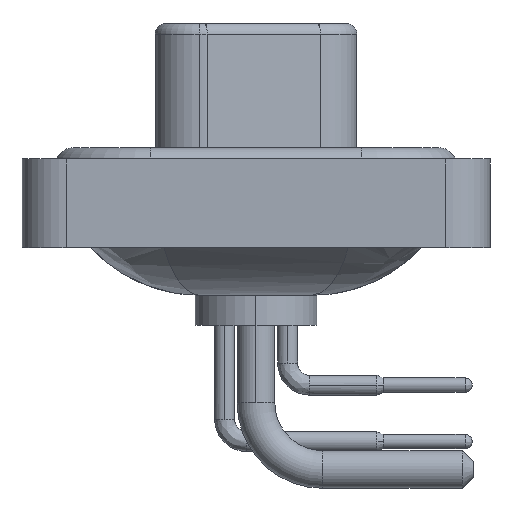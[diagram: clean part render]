
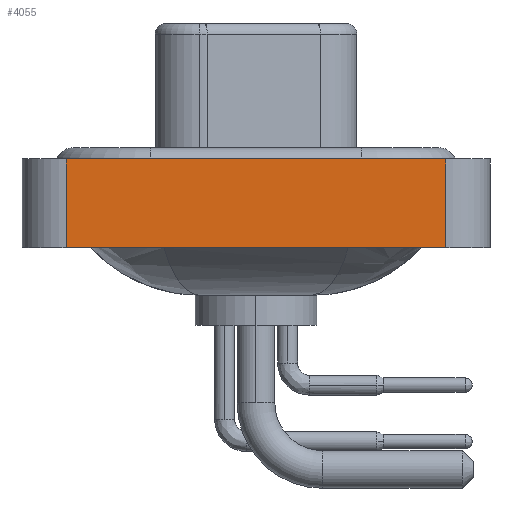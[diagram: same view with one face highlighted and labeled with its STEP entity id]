
A CAD part, left-side view. The second image highlights one B-rep face of the part: STEP entity #4055.
In plain terms, the highlighted planar face has unit normal (-1, 0, 0).
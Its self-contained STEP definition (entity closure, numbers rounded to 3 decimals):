
#981 = ORIENTED_EDGE ( 'NONE', *, *, #16964, .T. ) ;
#1514 = CARTESIAN_POINT ( 'NONE',  ( -7.35, -8.55, 0.4 ) ) ;
#2438 = ORIENTED_EDGE ( 'NONE', *, *, #9749, .F. ) ;
#3186 = AXIS2_PLACEMENT_3D ( 'NONE', #9276, #24573, #4792 ) ;
#3331 = DIRECTION ( 'NONE',  ( 0., 0., 1. ) ) ;
#3535 = EDGE_LOOP ( 'NONE', ( #981, #2438, #14370, #17733 ) ) ;
#4055 = ADVANCED_FACE ( 'NONE', ( #9128 ), #15759, .T. ) ;
#4123 = VECTOR ( 'NONE', #24071, 1000. ) ;
#4792 = DIRECTION ( 'NONE',  ( 0., 0., 1. ) ) ;
#4803 = EDGE_CURVE ( 'NONE', #16790, #16075, #14956, .T. ) ;
#5463 = CARTESIAN_POINT ( 'NONE',  ( -7.35, 8.55, -3.6 ) ) ;
#9128 = FACE_OUTER_BOUND ( 'NONE', #3535, .T. ) ;
#9276 = CARTESIAN_POINT ( 'NONE',  ( -7.35, -8.55, -3.6 ) ) ;
#9749 = EDGE_CURVE ( 'NONE', #14681, #9772, #12151, .T. ) ;
#9772 = VERTEX_POINT ( 'NONE', #11862 ) ;
#11862 = CARTESIAN_POINT ( 'NONE',  ( -7.35, -8.55, 0.4 ) ) ;
#12151 = LINE ( 'NONE', #1514, #17123 ) ;
#14370 = ORIENTED_EDGE ( 'NONE', *, *, #16257, .F. ) ;
#14681 = VERTEX_POINT ( 'NONE', #19489 ) ;
#14956 = LINE ( 'NONE', #15252, #4123 ) ;
#15029 = CARTESIAN_POINT ( 'NONE',  ( -7.35, -8.55, -3.6 ) ) ;
#15252 = CARTESIAN_POINT ( 'NONE',  ( -7.35, -8.55, -3.6 ) ) ;
#15508 = DIRECTION ( 'NONE',  ( 0., 0., 1. ) ) ;
#15759 = PLANE ( 'NONE',  #3186 ) ;
#16075 = VERTEX_POINT ( 'NONE', #15029 ) ;
#16257 = EDGE_CURVE ( 'NONE', #16790, #14681, #25246, .T. ) ;
#16790 = VERTEX_POINT ( 'NONE', #27802 ) ;
#16906 = DIRECTION ( 'NONE',  ( 0., -1., 0. ) ) ;
#16964 = EDGE_CURVE ( 'NONE', #16075, #9772, #26196, .T. ) ;
#17123 = VECTOR ( 'NONE', #16906, 1000. ) ;
#17733 = ORIENTED_EDGE ( 'NONE', *, *, #4803, .T. ) ;
#17964 = VECTOR ( 'NONE', #15508, 1000. ) ;
#19489 = CARTESIAN_POINT ( 'NONE',  ( -7.35, 8.55, 0.4 ) ) ;
#22984 = VECTOR ( 'NONE', #3331, 1000. ) ;
#24047 = CARTESIAN_POINT ( 'NONE',  ( -7.35, -8.55, -3.6 ) ) ;
#24071 = DIRECTION ( 'NONE',  ( 0., -1., 0. ) ) ;
#24573 = DIRECTION ( 'NONE',  ( -1., 0., 0. ) ) ;
#25246 = LINE ( 'NONE', #5463, #22984 ) ;
#26196 = LINE ( 'NONE', #24047, #17964 ) ;
#27802 = CARTESIAN_POINT ( 'NONE',  ( -7.35, 8.55, -3.6 ) ) ;
